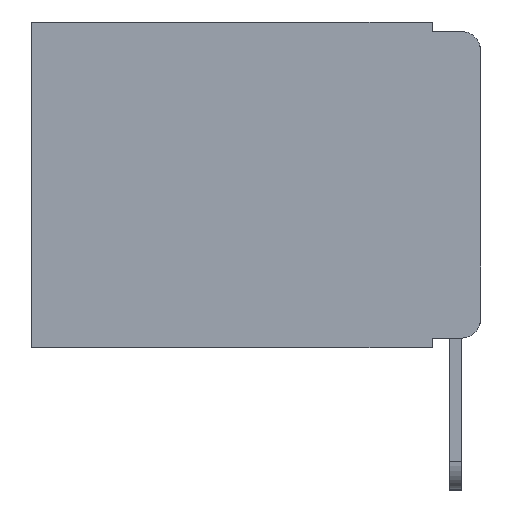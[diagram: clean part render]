
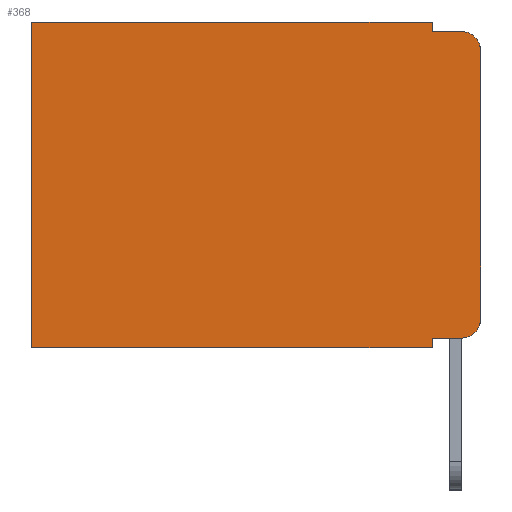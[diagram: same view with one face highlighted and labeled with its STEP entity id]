
A CAD part, left-side view. The second image highlights one B-rep face of the part: STEP entity #368.
In plain terms, the highlighted planar face has unit normal (-1, 0, 0).
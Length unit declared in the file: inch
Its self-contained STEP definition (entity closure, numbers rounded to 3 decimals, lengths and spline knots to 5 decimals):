
#85 = CARTESIAN_POINT ( 'NONE',  ( 0.298, 0.473, 0. ) ) ;
#233 = DIRECTION ( 'NONE',  ( 0., 0., -1. ) ) ;
#331 = VERTEX_POINT ( 'NONE', #3671 ) ;
#368 = ADVANCED_FACE ( 'NONE', ( #7433 ), #3950, .F. ) ;
#539 = AXIS2_PLACEMENT_3D ( 'NONE', #7250, #16471, #8672 ) ;
#831 = CARTESIAN_POINT ( 'NONE',  ( 0.298, 0., -0.313 ) ) ;
#964 = AXIS2_PLACEMENT_3D ( 'NONE', #6591, #9051, #16842 ) ;
#1151 = EDGE_CURVE ( 'NONE', #3597, #2509, #7826, .T. ) ;
#1169 = LINE ( 'NONE', #15496, #6883 ) ;
#1196 = ORIENTED_EDGE ( 'NONE', *, *, #11939, .T. ) ;
#1515 = ORIENTED_EDGE ( 'NONE', *, *, #6176, .T. ) ;
#1578 = EDGE_CURVE ( 'NONE', #3597, #15011, #4742, .T. ) ;
#1605 = DIRECTION ( 'NONE',  ( 0., 1., 0. ) ) ;
#1613 = DIRECTION ( 'NONE',  ( 0., 0., -1. ) ) ;
#1748 = CARTESIAN_POINT ( 'NONE',  ( 0.298, 0., -0.343 ) ) ;
#2248 = EDGE_CURVE ( 'NONE', #5594, #5008, #4068, .T. ) ;
#2448 = ORIENTED_EDGE ( 'NONE', *, *, #15709, .F. ) ;
#2509 = VERTEX_POINT ( 'NONE', #831 ) ;
#3017 = EDGE_CURVE ( 'NONE', #331, #9921, #14675, .T. ) ;
#3065 = DIRECTION ( 'NONE',  ( 0., 1., 0. ) ) ;
#3211 = CARTESIAN_POINT ( 'NONE',  ( 0.298, 0.473, 0. ) ) ;
#3597 = VERTEX_POINT ( 'NONE', #10306 ) ;
#3671 = CARTESIAN_POINT ( 'NONE',  ( 0.298, 0.051, -0.343 ) ) ;
#3750 = CARTESIAN_POINT ( 'NONE',  ( 0.298, 0.02, -0.333 ) ) ;
#3930 = CARTESIAN_POINT ( 'NONE',  ( 0.298, 0.473, -0.343 ) ) ;
#3950 = PLANE ( 'NONE',  #964 ) ;
#4068 = LINE ( 'NONE', #14541, #5494 ) ;
#4625 = AXIS2_PLACEMENT_3D ( 'NONE', #11459, #15422, #6399 ) ;
#4742 = CIRCLE ( 'NONE', #539, 0.02 ) ;
#5008 = VERTEX_POINT ( 'NONE', #9182 ) ;
#5258 = DIRECTION ( 'NONE',  ( 0., 0., -1. ) ) ;
#5494 = VECTOR ( 'NONE', #233, 39.37008 ) ;
#5594 = VERTEX_POINT ( 'NONE', #7831 ) ;
#5676 = VECTOR ( 'NONE', #8381, 39.37008 ) ;
#5741 = ORIENTED_EDGE ( 'NONE', *, *, #8383, .T. ) ;
#5807 = ORIENTED_EDGE ( 'NONE', *, *, #2248, .F. ) ;
#5927 = CARTESIAN_POINT ( 'NONE',  ( 0.298, 0.051, -0.333 ) ) ;
#5938 = CARTESIAN_POINT ( 'NONE',  ( 0.298, 0.02, -0.01 ) ) ;
#6133 = EDGE_LOOP ( 'NONE', ( #15069, #13804, #2448, #5807, #1196, #10955, #8543, #13426, #5741, #1515 ) ) ;
#6176 = EDGE_CURVE ( 'NONE', #8911, #2509, #9253, .T. ) ;
#6299 = VECTOR ( 'NONE', #3065, 39.37008 ) ;
#6399 = DIRECTION ( 'NONE',  ( 0., 0., -1. ) ) ;
#6591 = CARTESIAN_POINT ( 'NONE',  ( 0.298, 0., 0. ) ) ;
#6883 = VECTOR ( 'NONE', #8757, 39.37008 ) ;
#7079 = LINE ( 'NONE', #8985, #13820 ) ;
#7250 = CARTESIAN_POINT ( 'NONE',  ( 0.298, 0.02, -0.03 ) ) ;
#7330 = VECTOR ( 'NONE', #5258, 39.37008 ) ;
#7395 = LINE ( 'NONE', #9439, #7607 ) ;
#7433 = FACE_OUTER_BOUND ( 'NONE', #6133, .T. ) ;
#7607 = VECTOR ( 'NONE', #1605, 39.37008 ) ;
#7826 = LINE ( 'NONE', #9451, #9049 ) ;
#7831 = CARTESIAN_POINT ( 'NONE',  ( 0.298, 0.051, 0. ) ) ;
#8381 = DIRECTION ( 'NONE',  ( 0., -1., 0. ) ) ;
#8383 = EDGE_CURVE ( 'NONE', #11442, #8911, #11787, .T. ) ;
#8543 = ORIENTED_EDGE ( 'NONE', *, *, #3017, .F. ) ;
#8672 = DIRECTION ( 'NONE',  ( 0., 0., -1. ) ) ;
#8757 = DIRECTION ( 'NONE',  ( 0., 0., -1. ) ) ;
#8911 = VERTEX_POINT ( 'NONE', #3750 ) ;
#8985 = CARTESIAN_POINT ( 'NONE',  ( 0.298, 0.051, -0.01 ) ) ;
#9049 = VECTOR ( 'NONE', #1613, 39.37008 ) ;
#9051 = DIRECTION ( 'NONE',  ( 1., 0., 0. ) ) ;
#9182 = CARTESIAN_POINT ( 'NONE',  ( 0.298, 0.051, -0.01 ) ) ;
#9253 = CIRCLE ( 'NONE', #4625, 0.02 ) ;
#9439 = CARTESIAN_POINT ( 'NONE',  ( 0.298, 0., 0. ) ) ;
#9451 = CARTESIAN_POINT ( 'NONE',  ( 0.298, 0., 0. ) ) ;
#9921 = VERTEX_POINT ( 'NONE', #3930 ) ;
#10306 = CARTESIAN_POINT ( 'NONE',  ( 0.298, 0., -0.03 ) ) ;
#10955 = ORIENTED_EDGE ( 'NONE', *, *, #14773, .T. ) ;
#11442 = VERTEX_POINT ( 'NONE', #15272 ) ;
#11459 = CARTESIAN_POINT ( 'NONE',  ( 0.298, 0.02, -0.313 ) ) ;
#11787 = LINE ( 'NONE', #5927, #5676 ) ;
#11939 = EDGE_CURVE ( 'NONE', #5594, #13261, #7395, .T. ) ;
#12004 = LINE ( 'NONE', #85, #7330 ) ;
#13261 = VERTEX_POINT ( 'NONE', #3211 ) ;
#13426 = ORIENTED_EDGE ( 'NONE', *, *, #15785, .F. ) ;
#13804 = ORIENTED_EDGE ( 'NONE', *, *, #1578, .T. ) ;
#13820 = VECTOR ( 'NONE', #16624, 39.37008 ) ;
#14541 = CARTESIAN_POINT ( 'NONE',  ( 0.298, 0.051, 0. ) ) ;
#14675 = LINE ( 'NONE', #1748, #6299 ) ;
#14773 = EDGE_CURVE ( 'NONE', #13261, #9921, #12004, .T. ) ;
#15011 = VERTEX_POINT ( 'NONE', #5938 ) ;
#15069 = ORIENTED_EDGE ( 'NONE', *, *, #1151, .F. ) ;
#15272 = CARTESIAN_POINT ( 'NONE',  ( 0.298, 0.051, -0.333 ) ) ;
#15422 = DIRECTION ( 'NONE',  ( -1., 0., 0. ) ) ;
#15496 = CARTESIAN_POINT ( 'NONE',  ( 0.298, 0.051, 0. ) ) ;
#15709 = EDGE_CURVE ( 'NONE', #5008, #15011, #7079, .T. ) ;
#15785 = EDGE_CURVE ( 'NONE', #11442, #331, #1169, .T. ) ;
#16471 = DIRECTION ( 'NONE',  ( -1., 0., 0. ) ) ;
#16624 = DIRECTION ( 'NONE',  ( 0., -1., 0. ) ) ;
#16842 = DIRECTION ( 'NONE',  ( 0., 0., -1. ) ) ;
